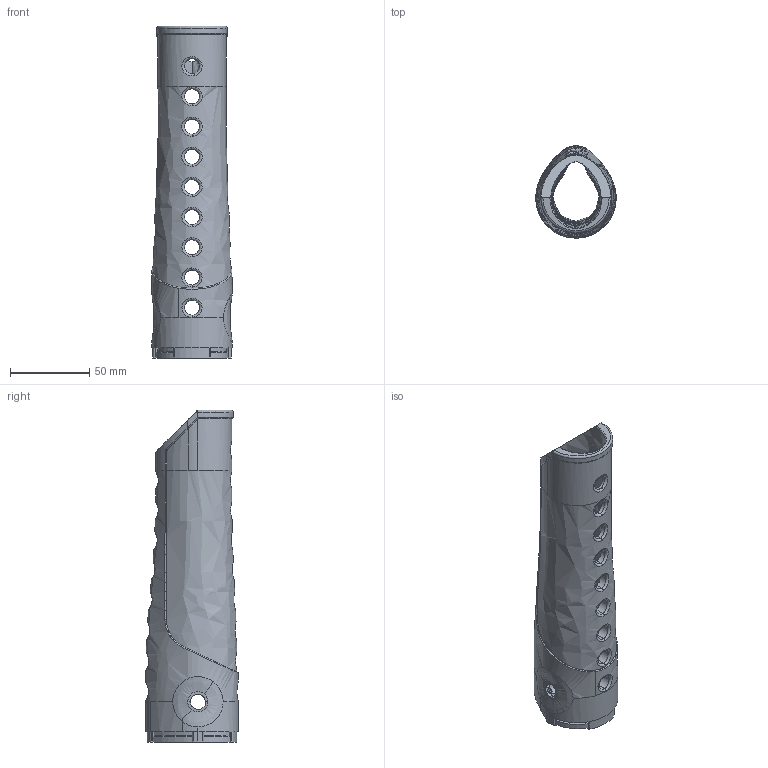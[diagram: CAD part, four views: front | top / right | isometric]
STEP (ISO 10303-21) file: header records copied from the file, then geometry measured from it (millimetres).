
FILE_DESCRIPTION (( 'STEP AP203' ), '1' );
FILE_NAME ('Orca Handguard Carbine V5.3.1.STEP', '2023-01-20T23:43:23', ( '' ), ( '' ), 'SwSTEP 2.0', 'SolidWorks 2021', '' );
FILE_SCHEMA (( 'CONFIG_CONTROL_DESIGN' ));
Products named in the file (1): Orca Handguard Carbine V5.3.1
Bounding box: 50.8 x 58.26 x 209.55 mm (x, y, z)
Volume: 183902.4 mm3; surface area: 56851.4 mm2
Topology: 1 solids, 1 shells, 342 faces, 1044 edges, 676 vertices
Faces by surface type: bspline 173, cylinder 79, plane 50, sphere 36, torus 4
Entity records: 38110 total; most frequent: CARTESIAN_POINT 30719, ORIENTED_EDGE 1944, EDGE_CURVE 972, DIRECTION 892, VERTEX_POINT 628, B_SPLINE_CURVE_WITH_KNOTS 579, EDGE_LOOP 378, ADVANCED_FACE 342
